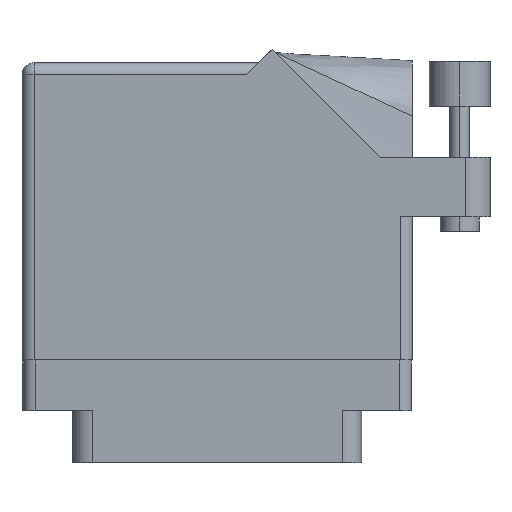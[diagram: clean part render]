
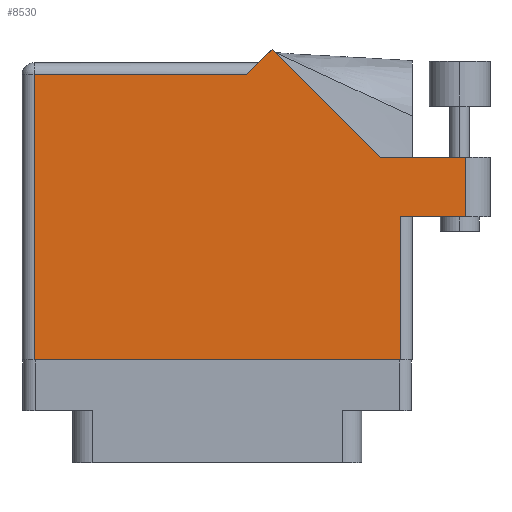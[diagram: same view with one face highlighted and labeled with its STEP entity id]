
A CAD part, front view. The second image highlights one B-rep face of the part: STEP entity #8530.
In plain terms, the highlighted face is planar.
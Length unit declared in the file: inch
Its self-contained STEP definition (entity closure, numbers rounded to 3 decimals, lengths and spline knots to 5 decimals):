
#598 = CARTESIAN_POINT ( 'NONE',  ( 1.84442, 1.044, 0. ) ) ;
#1273 = VECTOR ( 'NONE', #31208, 39.37008 ) ;
#3114 = CARTESIAN_POINT ( 'NONE',  ( 2.285, 0.737, 0. ) ) ;
#3129 = VERTEX_POINT ( 'NONE', #3114 ) ;
#3182 = CARTESIAN_POINT ( 'NONE',  ( 1.948, 0.737, 0. ) ) ;
#3739 = VERTEX_POINT ( 'NONE', #4042 ) ;
#4042 = CARTESIAN_POINT ( 'NONE',  ( 1.28771, 1.60071, 0. ) ) ;
#4225 = CARTESIAN_POINT ( 'NONE',  ( 2.285, 1.044, 0. ) ) ;
#4497 = VERTEX_POINT ( 'NONE', #12432 ) ;
#5304 = CARTESIAN_POINT ( 'NONE',  ( 0.062, 0., 0. ) ) ;
#5423 = ORIENTED_EDGE ( 'NONE', *, *, #19964, .T. ) ;
#5652 = DIRECTION ( 'NONE',  ( -0.707, 0.707, 0. ) ) ;
#5800 = DIRECTION ( 'NONE',  ( 0., 1., 0. ) ) ;
#6390 = EDGE_CURVE ( 'NONE', #29743, #34581, #28714, .T. ) ;
#6948 = VECTOR ( 'NONE', #10649, 39.37008 ) ;
#7031 = DIRECTION ( 'NONE',  ( 0., -1., 0. ) ) ;
#7235 = CARTESIAN_POINT ( 'NONE',  ( 2.285, 1.044, 0. ) ) ;
#7238 = EDGE_LOOP ( 'NONE', ( #34415, #8566, #12894, #14480, #5423, #22885, #14611, #26963, #7350 ) ) ;
#7329 = PLANE ( 'NONE',  #17686 ) ;
#7350 = ORIENTED_EDGE ( 'NONE', *, *, #6390, .T. ) ;
#7795 = CARTESIAN_POINT ( 'NONE',  ( 2.01, 0.737, 0. ) ) ;
#8412 = LINE ( 'NONE', #7235, #1273 ) ;
#8530 = ADVANCED_FACE ( 'NONE', ( #34929 ), #7329, .F. ) ;
#8566 = ORIENTED_EDGE ( 'NONE', *, *, #26262, .T. ) ;
#9507 = CARTESIAN_POINT ( 'NONE',  ( 0.062, 1.468, 0. ) ) ;
#9724 = EDGE_CURVE ( 'NONE', #4497, #3739, #27225, .T. ) ;
#9842 = CARTESIAN_POINT ( 'NONE',  ( 0., 1.53, 0. ) ) ;
#10116 = VECTOR ( 'NONE', #16224, 39.37008 ) ;
#10191 = DIRECTION ( 'NONE',  ( 0., 0., -1. ) ) ;
#10649 = DIRECTION ( 'NONE',  ( -0.707, -0.707, 0. ) ) ;
#10763 = CARTESIAN_POINT ( 'NONE',  ( 1.948, 0., 0. ) ) ;
#11291 = DIRECTION ( 'NONE',  ( -1., 0., 0. ) ) ;
#12432 = CARTESIAN_POINT ( 'NONE',  ( 1.84442, 1.044, 0. ) ) ;
#12451 = LINE ( 'NONE', #15589, #6948 ) ;
#12894 = ORIENTED_EDGE ( 'NONE', *, *, #18890, .T. ) ;
#14480 = ORIENTED_EDGE ( 'NONE', *, *, #9724, .T. ) ;
#14611 = ORIENTED_EDGE ( 'NONE', *, *, #28155, .T. ) ;
#14828 = VECTOR ( 'NONE', #7031, 39.37008 ) ;
#15273 = VERTEX_POINT ( 'NONE', #9507 ) ;
#15589 = CARTESIAN_POINT ( 'NONE',  ( 1.217, 1.53, 0. ) ) ;
#16224 = DIRECTION ( 'NONE',  ( 1., 0., 0. ) ) ;
#16845 = CARTESIAN_POINT ( 'NONE',  ( 2.41, 1.044, 0. ) ) ;
#17168 = EDGE_CURVE ( 'NONE', #25997, #29743, #27338, .T. ) ;
#17686 = AXIS2_PLACEMENT_3D ( 'NONE', #9842, #10191, #20692 ) ;
#17689 = CARTESIAN_POINT ( 'NONE',  ( 0.062, 0., 0. ) ) ;
#18857 = VECTOR ( 'NONE', #11291, 39.37008 ) ;
#18890 = EDGE_CURVE ( 'NONE', #30100, #4497, #31091, .T. ) ;
#19087 = CARTESIAN_POINT ( 'NONE',  ( 0., 0., 0. ) ) ;
#19964 = EDGE_CURVE ( 'NONE', #3739, #31065, #12451, .T. ) ;
#20692 = DIRECTION ( 'NONE',  ( -1., 0., 0. ) ) ;
#20733 = LINE ( 'NONE', #21519, #24083 ) ;
#21095 = VECTOR ( 'NONE', #5800, 39.37008 ) ;
#21519 = CARTESIAN_POINT ( 'NONE',  ( 0., 1.468, 0. ) ) ;
#21982 = LINE ( 'NONE', #17689, #14828 ) ;
#22885 = ORIENTED_EDGE ( 'NONE', *, *, #33778, .T. ) ;
#23980 = VECTOR ( 'NONE', #29152, 39.37008 ) ;
#24083 = VECTOR ( 'NONE', #29662, 39.37008 ) ;
#25997 = VERTEX_POINT ( 'NONE', #5304 ) ;
#26262 = EDGE_CURVE ( 'NONE', #3129, #30100, #8412, .T. ) ;
#26963 = ORIENTED_EDGE ( 'NONE', *, *, #17168, .T. ) ;
#27225 = LINE ( 'NONE', #598, #28941 ) ;
#27338 = LINE ( 'NONE', #19087, #10116 ) ;
#27975 = CARTESIAN_POINT ( 'NONE',  ( 1.948, 0.737, 0. ) ) ;
#28155 = EDGE_CURVE ( 'NONE', #15273, #25997, #21982, .T. ) ;
#28714 = LINE ( 'NONE', #3182, #21095 ) ;
#28941 = VECTOR ( 'NONE', #5652, 39.37008 ) ;
#29152 = DIRECTION ( 'NONE',  ( 1., 0., 0. ) ) ;
#29537 = EDGE_CURVE ( 'NONE', #34581, #3129, #32846, .T. ) ;
#29662 = DIRECTION ( 'NONE',  ( -1., 0., 0. ) ) ;
#29743 = VERTEX_POINT ( 'NONE', #10763 ) ;
#29986 = CARTESIAN_POINT ( 'NONE',  ( 1.155, 1.468, 0. ) ) ;
#30100 = VERTEX_POINT ( 'NONE', #4225 ) ;
#31065 = VERTEX_POINT ( 'NONE', #29986 ) ;
#31091 = LINE ( 'NONE', #16845, #18857 ) ;
#31208 = DIRECTION ( 'NONE',  ( 0., 1., 0. ) ) ;
#32846 = LINE ( 'NONE', #7795, #23980 ) ;
#33778 = EDGE_CURVE ( 'NONE', #31065, #15273, #20733, .T. ) ;
#34415 = ORIENTED_EDGE ( 'NONE', *, *, #29537, .T. ) ;
#34581 = VERTEX_POINT ( 'NONE', #27975 ) ;
#34929 = FACE_OUTER_BOUND ( 'NONE', #7238, .T. ) ;
